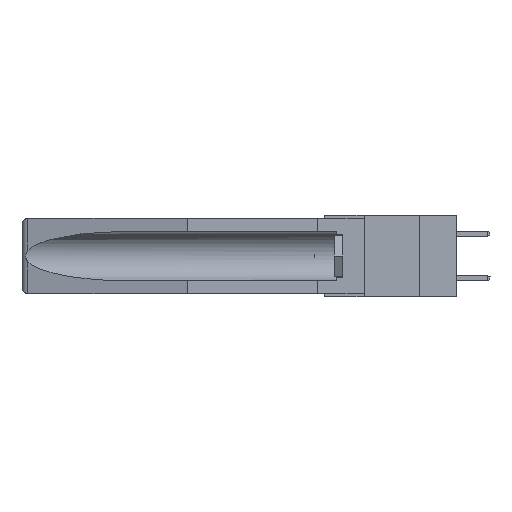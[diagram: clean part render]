
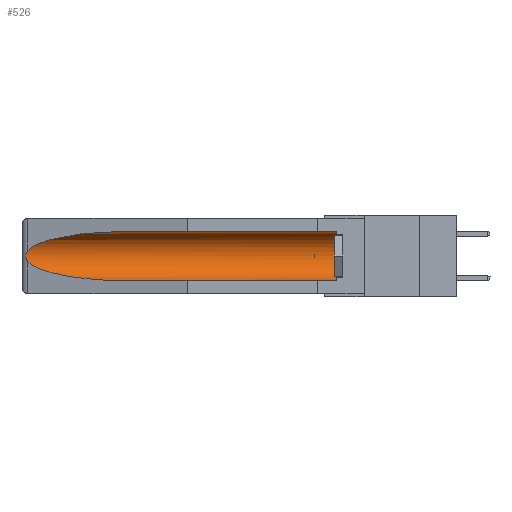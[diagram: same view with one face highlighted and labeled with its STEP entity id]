
A CAD part, left-side view. The second image highlights one B-rep face of the part: STEP entity #526.
In plain terms, the highlighted cylindrical face has radius 2.857 mm (diameter 5.715 mm), a partial arc.
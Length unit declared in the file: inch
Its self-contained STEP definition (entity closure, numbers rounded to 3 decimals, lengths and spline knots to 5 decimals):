
#526 = ADVANCED_FACE ( 'NONE', ( #11236 ), #25124, .F. ) ;
#615 = EDGE_CURVE ( 'NONE', #35782, #14925, #35630, .T. ) ;
#1041 = DIRECTION ( 'NONE',  ( 0., -1., 0. ) ) ;
#1132 = CARTESIAN_POINT ( 'NONE',  ( 0.155, 1.07973, -0.059 ) ) ;
#2309 = CARTESIAN_POINT ( 'NONE',  ( 0.155, 0.126, -0.284 ) ) ;
#2320 = LINE ( 'NONE', #31718, #4937 ) ;
#2808 = CARTESIAN_POINT ( 'NONE',  ( 0.26537, 1.52718, -0.14972 ) ) ;
#3428 = CARTESIAN_POINT ( 'NONE',  ( 0.26537, 1.52718, -0.19328 ) ) ;
#3682 = AXIS2_PLACEMENT_3D ( 'NONE', #7984, #32693, #19033 ) ;
#3916 = EDGE_CURVE ( 'NONE', #24242, #26172, #22778, .T. ) ;
#4937 = VECTOR ( 'NONE', #28708, 39.37008 ) ;
#6106 = CARTESIAN_POINT ( 'NONE',  ( 0.21114, 1.30732, -0.284 ) ) ;
#7099 = EDGE_CURVE ( 'NONE', #23513, #35782, #19538, .T. ) ;
#7984 = CARTESIAN_POINT ( 'NONE',  ( 0.155, -0.30754, -0.1715 ) ) ;
#8110 = CARTESIAN_POINT ( 'NONE',  ( 0.26537, 1.52718, -0.14972 ) ) ;
#9466 = CARTESIAN_POINT ( 'NONE',  ( 0.2673, 1.5327, -0.16383 ) ) ;
#9965 = CARTESIAN_POINT ( 'NONE',  ( 0.2675, 1.53308, -0.17534 ) ) ;
#10828 = AXIS2_PLACEMENT_3D ( 'NONE', #31666, #1041, #20295 ) ;
#11236 = FACE_OUTER_BOUND ( 'NONE', #13189, .T. ) ;
#12322 = ORIENTED_EDGE ( 'NONE', *, *, #3916, .T. ) ;
#12804 = ORIENTED_EDGE ( 'NONE', *, *, #615, .T. ) ;
#13189 = EDGE_LOOP ( 'NONE', ( #12804, #32544, #12322, #16015, #14518, #29159 ) ) ;
#14518 = ORIENTED_EDGE ( 'NONE', *, *, #33551, .T. ) ;
#14925 = VERTEX_POINT ( 'NONE', #2808 ) ;
#15054 = CARTESIAN_POINT ( 'NONE',  ( 0.26654, 1.53092, -0.15636 ) ) ;
#15186 = CARTESIAN_POINT ( 'NONE',  ( 0.26597, 1.5296, -0.19026 ) ) ;
#15363 = B_SPLINE_CURVE_WITH_KNOTS ( 'NONE', 3,
 ( #34642, #26073, #15054, #9466, #28974, #9965, #23563, #18095, #15186, #31989 ),
 .UNSPECIFIED., .F., .F.,
 ( 4, 2, 2, 2, 4 ),
 ( 0., 0.00029, 0.00058, 0.00087, 0.00117 ),
 .UNSPECIFIED. ) ;
#16015 = ORIENTED_EDGE ( 'NONE', *, *, #23413, .F. ) ;
#18095 = CARTESIAN_POINT ( 'NONE',  ( 0.26655, 1.53094, -0.18657 ) ) ;
#18506 = CIRCLE ( 'NONE', #10828, 0.1125 ) ;
#19033 = DIRECTION ( 'NONE',  ( 0., 0., 1. ) ) ;
#19403 = CARTESIAN_POINT ( 'NONE',  ( 0.155, 1.07973, -0.059 ) ) ;
#19538 = LINE ( 'NONE', #32259, #33797 ) ;
#20295 = DIRECTION ( 'NONE',  ( 0., 0., 1. ) ) ;
#21024 = CARTESIAN_POINT ( 'NONE',  ( 0.26537, 1.52718, -0.19328 ) ) ;
#22040 = CARTESIAN_POINT ( 'NONE',  ( 0.25451, 1.48313, -0.09465 ) ) ;
#22778 =( BOUNDED_CURVE ( )  B_SPLINE_CURVE ( 3, ( #3428, #22955, #6106, #33826 ),
 .UNSPECIFIED., .F., .F. ) 
 B_SPLINE_CURVE_WITH_KNOTS ( ( 4, 4 ),
 ( 0.1948, 1.5708 ),
 .UNSPECIFIED. ) 
 CURVE ( )  GEOMETRIC_REPRESENTATION_ITEM ( )  RATIONAL_B_SPLINE_CURVE ( ( 1., 0.848, 0.848, 1. ) ) 
 REPRESENTATION_ITEM ( '' )  );
#22855 = EDGE_CURVE ( 'NONE', #14925, #24242, #15363, .T. ) ;
#22955 = CARTESIAN_POINT ( 'NONE',  ( 0.25451, 1.48313, -0.24835 ) ) ;
#22975 = VERTEX_POINT ( 'NONE', #2309 ) ;
#23029 = CARTESIAN_POINT ( 'NONE',  ( 0.155, 0.126, -0.059 ) ) ;
#23413 = EDGE_CURVE ( 'NONE', #22975, #26172, #2320, .T. ) ;
#23513 = VERTEX_POINT ( 'NONE', #23029 ) ;
#23563 = CARTESIAN_POINT ( 'NONE',  ( 0.2673, 1.53269, -0.17917 ) ) ;
#24242 = VERTEX_POINT ( 'NONE', #21024 ) ;
#25124 = CYLINDRICAL_SURFACE ( 'NONE', #3682, 0.1125 ) ;
#26073 = CARTESIAN_POINT ( 'NONE',  ( 0.26597, 1.52961, -0.15275 ) ) ;
#26172 = VERTEX_POINT ( 'NONE', #33015 ) ;
#26973 = DIRECTION ( 'NONE',  ( 0., 1., 0. ) ) ;
#28708 = DIRECTION ( 'NONE',  ( 0., 1., 0. ) ) ;
#28974 = CARTESIAN_POINT ( 'NONE',  ( 0.2675, 1.53308, -0.16763 ) ) ;
#29159 = ORIENTED_EDGE ( 'NONE', *, *, #7099, .T. ) ;
#30749 = CARTESIAN_POINT ( 'NONE',  ( 0.21114, 1.30732, -0.059 ) ) ;
#31666 = CARTESIAN_POINT ( 'NONE',  ( 0.155, 0.126, -0.1715 ) ) ;
#31718 = CARTESIAN_POINT ( 'NONE',  ( 0.155, -0.30754, -0.284 ) ) ;
#31989 = CARTESIAN_POINT ( 'NONE',  ( 0.26537, 1.52718, -0.19328 ) ) ;
#32259 = CARTESIAN_POINT ( 'NONE',  ( 0.155, -0.30754, -0.059 ) ) ;
#32544 = ORIENTED_EDGE ( 'NONE', *, *, #22855, .T. ) ;
#32693 = DIRECTION ( 'NONE',  ( 0., 1., 0. ) ) ;
#33015 = CARTESIAN_POINT ( 'NONE',  ( 0.155, 1.07973, -0.284 ) ) ;
#33551 = EDGE_CURVE ( 'NONE', #22975, #23513, #18506, .T. ) ;
#33797 = VECTOR ( 'NONE', #26973, 39.37008 ) ;
#33826 = CARTESIAN_POINT ( 'NONE',  ( 0.155, 1.07973, -0.284 ) ) ;
#34642 = CARTESIAN_POINT ( 'NONE',  ( 0.26537, 1.52718, -0.14972 ) ) ;
#35630 =( BOUNDED_CURVE ( )  B_SPLINE_CURVE ( 3, ( #19403, #30749, #22040, #8110 ),
 .UNSPECIFIED., .F., .F. ) 
 B_SPLINE_CURVE_WITH_KNOTS ( ( 4, 4 ),
 ( 4.71239, 6.08839 ),
 .UNSPECIFIED. ) 
 CURVE ( )  GEOMETRIC_REPRESENTATION_ITEM ( )  RATIONAL_B_SPLINE_CURVE ( ( 1., 0.848, 0.848, 1. ) ) 
 REPRESENTATION_ITEM ( '' )  );
#35782 = VERTEX_POINT ( 'NONE', #1132 ) ;
